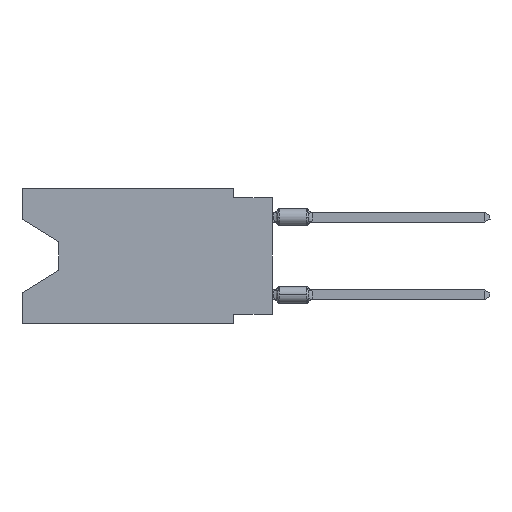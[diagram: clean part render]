
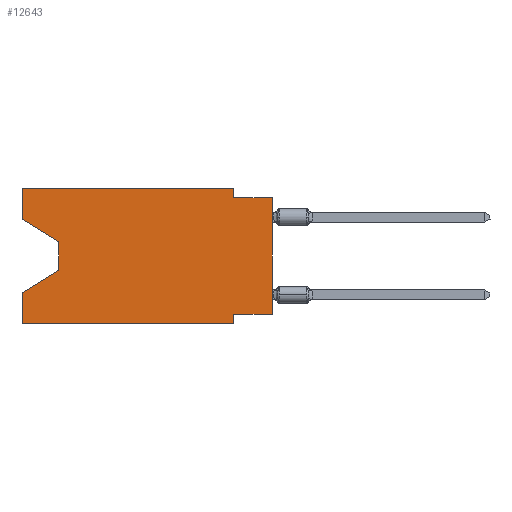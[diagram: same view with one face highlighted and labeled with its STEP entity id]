
A CAD part, left-side view. The second image highlights one B-rep face of the part: STEP entity #12643.
In plain terms, the highlighted planar face has unit normal (-1, 0, 0).
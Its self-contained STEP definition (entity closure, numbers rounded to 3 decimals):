
#30 = VERTEX_POINT ( 'NONE', #5017 ) ;
#1880 = LINE ( 'NONE', #15374, #14259 ) ;
#1945 = LINE ( 'NONE', #36969, #30049 ) ;
#1954 = CARTESIAN_POINT ( 'NONE',  ( 0., 16.383, 0. ) ) ;
#2220 = LINE ( 'NONE', #1954, #7302 ) ;
#2304 = DIRECTION ( 'NONE',  ( 0., -1., 0. ) ) ;
#2520 = DIRECTION ( 'NONE',  ( 0., 0., -1. ) ) ;
#2595 = VECTOR ( 'NONE', #25436, 1000. ) ;
#3380 = VECTOR ( 'NONE', #46452, 1000. ) ;
#4368 = VECTOR ( 'NONE', #2304, 1000. ) ;
#4724 = EDGE_CURVE ( 'NONE', #10089, #29342, #25824, .T. ) ;
#5017 = CARTESIAN_POINT ( 'NONE',  ( 0., 16.383, -8.89 ) ) ;
#5119 = VECTOR ( 'NONE', #14989, 1000. ) ;
#5821 = LINE ( 'NONE', #44334, #50676 ) ;
#6506 = ORIENTED_EDGE ( 'NONE', *, *, #4724, .F. ) ;
#7302 = VECTOR ( 'NONE', #46483, 1000. ) ;
#7834 = DIRECTION ( 'NONE',  ( 0., 0., -1. ) ) ;
#7915 = LINE ( 'NONE', #21397, #2595 ) ;
#8131 = EDGE_CURVE ( 'NONE', #17796, #10089, #40728, .T. ) ;
#8193 = CARTESIAN_POINT ( 'NONE',  ( 0., 13.97, -5.385 ) ) ;
#8698 = ORIENTED_EDGE ( 'NONE', *, *, #51761, .T. ) ;
#9795 = CARTESIAN_POINT ( 'NONE',  ( 0., 16.383, -8.89 ) ) ;
#10089 = VERTEX_POINT ( 'NONE', #37325 ) ;
#10243 = ORIENTED_EDGE ( 'NONE', *, *, #37216, .T. ) ;
#10373 = CARTESIAN_POINT ( 'NONE',  ( 0., 2.54, -8.89 ) ) ;
#11374 = LINE ( 'NONE', #28895, #3380 ) ;
#12643 = ADVANCED_FACE ( 'NONE', ( #33675 ), #34225, .F. ) ;
#14259 = VECTOR ( 'NONE', #14799, 1000. ) ;
#14580 = VECTOR ( 'NONE', #28417, 1000. ) ;
#14799 = DIRECTION ( 'NONE',  ( 0., 0., 1. ) ) ;
#14989 = DIRECTION ( 'NONE',  ( 0., -1., 0. ) ) ;
#15374 = CARTESIAN_POINT ( 'NONE',  ( 0., 16.383, 0. ) ) ;
#16470 = DIRECTION ( 'NONE',  ( 1., 0., 0. ) ) ;
#16803 = EDGE_CURVE ( 'NONE', #23299, #21621, #5821, .T. ) ;
#17001 = CARTESIAN_POINT ( 'NONE',  ( 0., 16.383, 0. ) ) ;
#17234 = ORIENTED_EDGE ( 'NONE', *, *, #47613, .T. ) ;
#17472 = ORIENTED_EDGE ( 'NONE', *, *, #16803, .T. ) ;
#17796 = VERTEX_POINT ( 'NONE', #41514 ) ;
#18345 = DIRECTION ( 'NONE',  ( 0., 0., -1. ) ) ;
#19508 = LINE ( 'NONE', #28687, #30147 ) ;
#19514 = VERTEX_POINT ( 'NONE', #28803 ) ;
#19794 = LINE ( 'NONE', #53737, #14580 ) ;
#20110 = DIRECTION ( 'NONE',  ( 0., -0.855, -0.519 ) ) ;
#20393 = CARTESIAN_POINT ( 'NONE',  ( 0., 16.383, 0. ) ) ;
#21311 = CARTESIAN_POINT ( 'NONE',  ( 0., 0., -8.255 ) ) ;
#21397 = CARTESIAN_POINT ( 'NONE',  ( 0., 2.54, -8.89 ) ) ;
#21621 = VERTEX_POINT ( 'NONE', #42712 ) ;
#22353 = CARTESIAN_POINT ( 'NONE',  ( 0., 13.97, -3.505 ) ) ;
#23299 = VERTEX_POINT ( 'NONE', #8193 ) ;
#23846 = VERTEX_POINT ( 'NONE', #22353 ) ;
#24929 = EDGE_CURVE ( 'NONE', #29393, #30718, #19794, .T. ) ;
#25436 = DIRECTION ( 'NONE',  ( 0., 0., -1. ) ) ;
#25612 = EDGE_CURVE ( 'NONE', #30, #21621, #2220, .T. ) ;
#25824 = LINE ( 'NONE', #43347, #36441 ) ;
#26002 = EDGE_LOOP ( 'NONE', ( #8698, #46729, #17472, #40194, #17234, #26889, #52424, #10243, #6506, #34117, #49269, #42400 ) ) ;
#26889 = ORIENTED_EDGE ( 'NONE', *, *, #31841, .F. ) ;
#28194 = VERTEX_POINT ( 'NONE', #47133 ) ;
#28417 = DIRECTION ( 'NONE',  ( 0., 1., 0. ) ) ;
#28687 = CARTESIAN_POINT ( 'NONE',  ( 0., 16.383, -2.038 ) ) ;
#28803 = CARTESIAN_POINT ( 'NONE',  ( 0., 16.383, -2.038 ) ) ;
#28895 = CARTESIAN_POINT ( 'NONE',  ( 0., 0., 0. ) ) ;
#29293 = VECTOR ( 'NONE', #18345, 1000. ) ;
#29342 = VERTEX_POINT ( 'NONE', #37966 ) ;
#29393 = VERTEX_POINT ( 'NONE', #21311 ) ;
#30049 = VECTOR ( 'NONE', #2520, 1000. ) ;
#30147 = VECTOR ( 'NONE', #20110, 1000. ) ;
#30718 = VERTEX_POINT ( 'NONE', #51029 ) ;
#31841 = EDGE_CURVE ( 'NONE', #30718, #41602, #7915, .T. ) ;
#33577 = LINE ( 'NONE', #20393, #5119 ) ;
#33675 = FACE_OUTER_BOUND ( 'NONE', #26002, .T. ) ;
#34117 = ORIENTED_EDGE ( 'NONE', *, *, #8131, .F. ) ;
#34225 = PLANE ( 'NONE',  #51011 ) ;
#36441 = VECTOR ( 'NONE', #56602, 1000. ) ;
#36969 = CARTESIAN_POINT ( 'NONE',  ( 0., 13.97, -3.505 ) ) ;
#37216 = EDGE_CURVE ( 'NONE', #29393, #29342, #11374, .T. ) ;
#37325 = CARTESIAN_POINT ( 'NONE',  ( 0., 2.54, -0.635 ) ) ;
#37966 = CARTESIAN_POINT ( 'NONE',  ( 0., 0., -0.635 ) ) ;
#40074 = EDGE_CURVE ( 'NONE', #23846, #23299, #1945, .T. ) ;
#40194 = ORIENTED_EDGE ( 'NONE', *, *, #25612, .F. ) ;
#40728 = LINE ( 'NONE', #53697, #29293 ) ;
#41165 = DIRECTION ( 'NONE',  ( 0., 0.855, -0.519 ) ) ;
#41514 = CARTESIAN_POINT ( 'NONE',  ( 0., 2.54, 0. ) ) ;
#41602 = VERTEX_POINT ( 'NONE', #10373 ) ;
#41648 = LINE ( 'NONE', #9795, #4368 ) ;
#42400 = ORIENTED_EDGE ( 'NONE', *, *, #45540, .F. ) ;
#42712 = CARTESIAN_POINT ( 'NONE',  ( 0., 16.383, -6.852 ) ) ;
#43347 = CARTESIAN_POINT ( 'NONE',  ( 0., 0., -0.635 ) ) ;
#44334 = CARTESIAN_POINT ( 'NONE',  ( 0., 13.97, -5.385 ) ) ;
#45540 = EDGE_CURVE ( 'NONE', #19514, #28194, #1880, .T. ) ;
#46452 = DIRECTION ( 'NONE',  ( 0., 0., 1. ) ) ;
#46483 = DIRECTION ( 'NONE',  ( 0., 0., 1. ) ) ;
#46729 = ORIENTED_EDGE ( 'NONE', *, *, #40074, .T. ) ;
#47133 = CARTESIAN_POINT ( 'NONE',  ( 0., 16.383, 0. ) ) ;
#47613 = EDGE_CURVE ( 'NONE', #30, #41602, #41648, .T. ) ;
#48675 = EDGE_CURVE ( 'NONE', #28194, #17796, #33577, .T. ) ;
#49269 = ORIENTED_EDGE ( 'NONE', *, *, #48675, .F. ) ;
#50676 = VECTOR ( 'NONE', #41165, 1000. ) ;
#51011 = AXIS2_PLACEMENT_3D ( 'NONE', #17001, #16470, #7834 ) ;
#51029 = CARTESIAN_POINT ( 'NONE',  ( 0., 2.54, -8.255 ) ) ;
#51761 = EDGE_CURVE ( 'NONE', #19514, #23846, #19508, .T. ) ;
#52424 = ORIENTED_EDGE ( 'NONE', *, *, #24929, .F. ) ;
#53697 = CARTESIAN_POINT ( 'NONE',  ( 0., 2.54, 0. ) ) ;
#53737 = CARTESIAN_POINT ( 'NONE',  ( 0., 0., -8.255 ) ) ;
#56602 = DIRECTION ( 'NONE',  ( 0., -1., 0. ) ) ;
